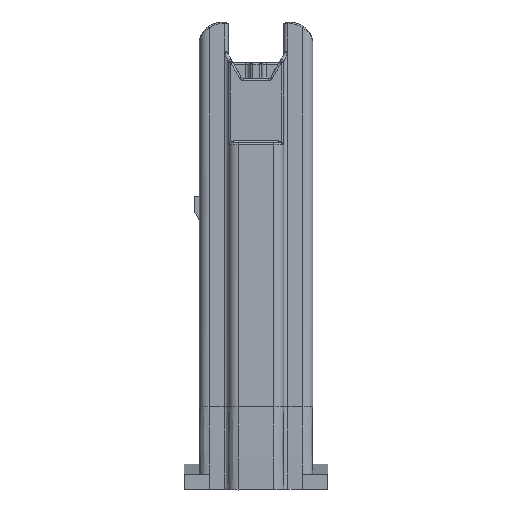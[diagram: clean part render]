
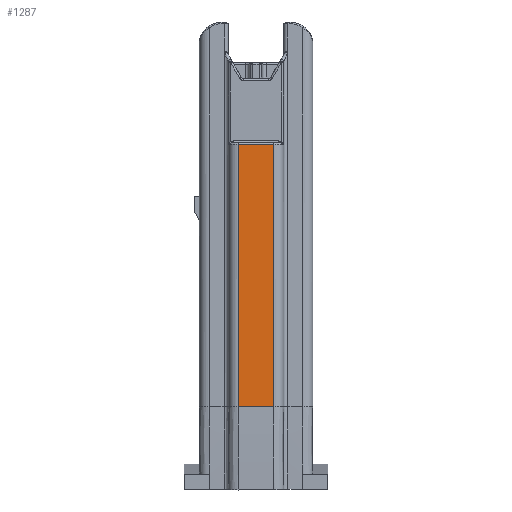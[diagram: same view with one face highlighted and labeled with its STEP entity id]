
A CAD part, top view. The second image highlights one B-rep face of the part: STEP entity #1287.
In plain terms, the highlighted planar face has unit normal (0, 0, 1).
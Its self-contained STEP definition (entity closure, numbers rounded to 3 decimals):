
#107 = EDGE_CURVE ( 'NONE', #12285, #4871, #2760, .T. ) ;
#466 = LINE ( 'NONE', #1599, #11120 ) ;
#1287 = ADVANCED_FACE ( 'NONE', ( #2587 ), #13256, .F. ) ;
#1599 = CARTESIAN_POINT ( 'NONE',  ( 3.531, 26.01, 34.163 ) ) ;
#2006 = ORIENTED_EDGE ( 'NONE', *, *, #2007, .F. ) ;
#2007 = EDGE_CURVE ( 'NONE', #12974, #9126, #466, .T. ) ;
#2284 = DIRECTION ( 'NONE',  ( 1., 0., 0. ) ) ;
#2587 = FACE_OUTER_BOUND ( 'NONE', #4713, .T. ) ;
#2760 = LINE ( 'NONE', #5131, #8256 ) ;
#3006 = CARTESIAN_POINT ( 'NONE',  ( 3.531, 0., 34.163 ) ) ;
#3098 = ORIENTED_EDGE ( 'NONE', *, *, #10223, .T. ) ;
#3258 = CARTESIAN_POINT ( 'NONE',  ( 3.531, 52.019, 34.163 ) ) ;
#3336 = CARTESIAN_POINT ( 'NONE',  ( 0., 52.019, 34.163 ) ) ;
#3512 = DIRECTION ( 'NONE',  ( 0., 0., -1. ) ) ;
#4713 = EDGE_LOOP ( 'NONE', ( #2006, #7186, #10682, #3098 ) ) ;
#4871 = VERTEX_POINT ( 'NONE', #7158 ) ;
#5131 = CARTESIAN_POINT ( 'NONE',  ( -3.531, 34.419, 34.163 ) ) ;
#5274 = CARTESIAN_POINT ( 'NONE',  ( -3.531, 52.019, 34.163 ) ) ;
#5378 = VECTOR ( 'NONE', #2284, 1000. ) ;
#5697 = LINE ( 'NONE', #9110, #11508 ) ;
#6118 = DIRECTION ( 'NONE',  ( 1., 0., 0. ) ) ;
#7158 = CARTESIAN_POINT ( 'NONE',  ( -3.531, 0., 34.163 ) ) ;
#7186 = ORIENTED_EDGE ( 'NONE', *, *, #9441, .F. ) ;
#7462 = DIRECTION ( 'NONE',  ( 0., -1., 0. ) ) ;
#7565 = CARTESIAN_POINT ( 'NONE',  ( 3.531, 0., 34.163 ) ) ;
#8256 = VECTOR ( 'NONE', #7462, 1000. ) ;
#9110 = CARTESIAN_POINT ( 'NONE',  ( 0., 0., 34.163 ) ) ;
#9126 = VERTEX_POINT ( 'NONE', #7565 ) ;
#9440 = AXIS2_PLACEMENT_3D ( 'NONE', #3006, #3512, #10701 ) ;
#9441 = EDGE_CURVE ( 'NONE', #12285, #12974, #10865, .T. ) ;
#10223 = EDGE_CURVE ( 'NONE', #4871, #9126, #5697, .T. ) ;
#10682 = ORIENTED_EDGE ( 'NONE', *, *, #107, .T. ) ;
#10701 = DIRECTION ( 'NONE',  ( -1., 0., 0. ) ) ;
#10865 = LINE ( 'NONE', #3336, #5378 ) ;
#11120 = VECTOR ( 'NONE', #12937, 1000. ) ;
#11508 = VECTOR ( 'NONE', #6118, 1000. ) ;
#12285 = VERTEX_POINT ( 'NONE', #5274 ) ;
#12937 = DIRECTION ( 'NONE',  ( 0., -1., 0. ) ) ;
#12974 = VERTEX_POINT ( 'NONE', #3258 ) ;
#13256 = PLANE ( 'NONE',  #9440 ) ;
